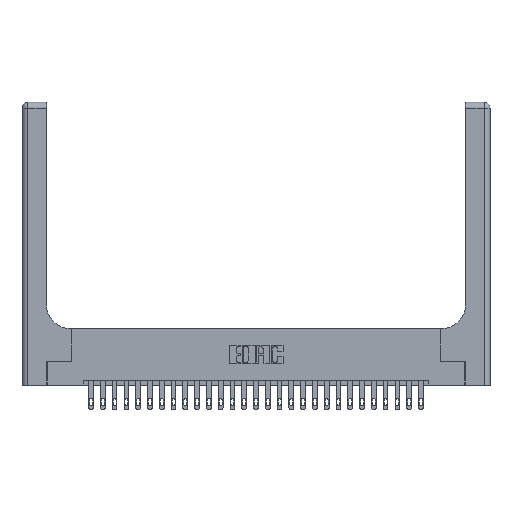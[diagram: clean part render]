
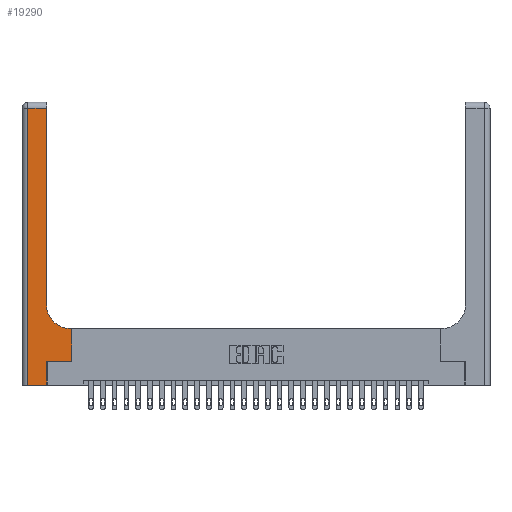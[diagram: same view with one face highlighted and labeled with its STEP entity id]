
A CAD part, top view. The second image highlights one B-rep face of the part: STEP entity #19290.
In plain terms, the highlighted planar face has unit normal (0, 0, 1).
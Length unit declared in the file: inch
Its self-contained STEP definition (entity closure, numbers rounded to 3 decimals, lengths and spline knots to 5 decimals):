
#287 = DIRECTION ( 'NONE',  ( 0., 0., -1. ) ) ;
#476 = EDGE_CURVE ( 'NONE', #22405, #22920, #10577, .T. ) ;
#530 = DIRECTION ( 'NONE',  ( 0., -1., 0. ) ) ;
#1336 = VERTEX_POINT ( 'NONE', #18872 ) ;
#1793 = VERTEX_POINT ( 'NONE', #12462 ) ;
#2691 = VECTOR ( 'NONE', #4734, 39.37008 ) ;
#3200 = CARTESIAN_POINT ( 'NONE',  ( 0.265, 0.25, 0.37 ) ) ;
#4323 = VECTOR ( 'NONE', #20410, 39.37008 ) ;
#4428 = LINE ( 'NONE', #23017, #19224 ) ;
#4638 = DIRECTION ( 'NONE',  ( -1., 0., 0. ) ) ;
#4734 = DIRECTION ( 'NONE',  ( 1., 0., 0. ) ) ;
#4810 = DIRECTION ( 'NONE',  ( -1., 0., 0. ) ) ;
#5131 = VECTOR ( 'NONE', #22413, 39.37008 ) ;
#5267 = EDGE_LOOP ( 'NONE', ( #17801, #13367, #9444, #25422, #22040, #21015, #5720, #16554, #16107 ) ) ;
#5720 = ORIENTED_EDGE ( 'NONE', *, *, #18563, .T. ) ;
#5885 = CARTESIAN_POINT ( 'NONE',  ( 0.51, 0.6, 0.37 ) ) ;
#6040 = DIRECTION ( 'NONE',  ( 0., 1., 0. ) ) ;
#6637 = PLANE ( 'NONE',  #23542 ) ;
#6840 = DIRECTION ( 'NONE',  ( 1., 0., 0. ) ) ;
#7243 = CARTESIAN_POINT ( 'NONE',  ( 0.265, 0.25, 0.37 ) ) ;
#8578 = CARTESIAN_POINT ( 'NONE',  ( 0., 2.94, 0.37 ) ) ;
#8591 = VECTOR ( 'NONE', #530, 39.37008 ) ;
#9444 = ORIENTED_EDGE ( 'NONE', *, *, #16379, .T. ) ;
#10037 = LINE ( 'NONE', #16149, #11757 ) ;
#10207 = AXIS2_PLACEMENT_3D ( 'NONE', #25192, #25063, #6840 ) ;
#10384 = VERTEX_POINT ( 'NONE', #10520 ) ;
#10520 = CARTESIAN_POINT ( 'NONE',  ( 0.06, 0., 0.37 ) ) ;
#10577 = LINE ( 'NONE', #8578, #4323 ) ;
#11757 = VECTOR ( 'NONE', #6040, 39.37008 ) ;
#11845 = VERTEX_POINT ( 'NONE', #3200 ) ;
#12185 = CARTESIAN_POINT ( 'NONE',  ( 0.26, 3., 0.37 ) ) ;
#12462 = CARTESIAN_POINT ( 'NONE',  ( 0.265, 0., 0.37 ) ) ;
#12566 = EDGE_CURVE ( 'NONE', #23044, #22405, #18050, .T. ) ;
#12725 = CARTESIAN_POINT ( 'NONE',  ( 0.06, 2.94, 0.37 ) ) ;
#12739 = LINE ( 'NONE', #14986, #8591 ) ;
#12757 = EDGE_CURVE ( 'NONE', #25190, #23044, #21658, .T. ) ;
#13367 = ORIENTED_EDGE ( 'NONE', *, *, #476, .T. ) ;
#14268 = VECTOR ( 'NONE', #16799, 39.37008 ) ;
#14986 = CARTESIAN_POINT ( 'NONE',  ( 0.06, 3., 0.37 ) ) ;
#15117 = LINE ( 'NONE', #7243, #2691 ) ;
#15426 = EDGE_CURVE ( 'NONE', #11845, #1336, #15117, .T. ) ;
#16107 = ORIENTED_EDGE ( 'NONE', *, *, #12757, .T. ) ;
#16149 = CARTESIAN_POINT ( 'NONE',  ( 0.265, 0., 0.37 ) ) ;
#16379 = EDGE_CURVE ( 'NONE', #22920, #10384, #12739, .T. ) ;
#16554 = ORIENTED_EDGE ( 'NONE', *, *, #17164, .T. ) ;
#16799 = DIRECTION ( 'NONE',  ( 1., 0., 0. ) ) ;
#17164 = EDGE_CURVE ( 'NONE', #21154, #25190, #4428, .T. ) ;
#17166 = VECTOR ( 'NONE', #21677, 39.37008 ) ;
#17801 = ORIENTED_EDGE ( 'NONE', *, *, #12566, .T. ) ;
#18050 = LINE ( 'NONE', #12185, #5131 ) ;
#18563 = EDGE_CURVE ( 'NONE', #1336, #21154, #21427, .T. ) ;
#18615 = CARTESIAN_POINT ( 'NONE',  ( 0.26, 2.94, 0.37 ) ) ;
#18872 = CARTESIAN_POINT ( 'NONE',  ( 0.528, 0.25, 0.37 ) ) ;
#19224 = VECTOR ( 'NONE', #4810, 39.37008 ) ;
#19290 = ADVANCED_FACE ( 'NONE', ( #24841 ), #6637, .F. ) ;
#20362 = EDGE_CURVE ( 'NONE', #10384, #1793, #24509, .T. ) ;
#20410 = DIRECTION ( 'NONE',  ( -1., 0., 0. ) ) ;
#20441 = CARTESIAN_POINT ( 'NONE',  ( 0.528, 0.6, 0.37 ) ) ;
#21015 = ORIENTED_EDGE ( 'NONE', *, *, #15426, .T. ) ;
#21154 = VERTEX_POINT ( 'NONE', #20441 ) ;
#21427 = LINE ( 'NONE', #25695, #17166 ) ;
#21658 = CIRCLE ( 'NONE', #10207, 0.25 ) ;
#21677 = DIRECTION ( 'NONE',  ( 0., 1., 0. ) ) ;
#22040 = ORIENTED_EDGE ( 'NONE', *, *, #23774, .T. ) ;
#22405 = VERTEX_POINT ( 'NONE', #18615 ) ;
#22413 = DIRECTION ( 'NONE',  ( 0., 1., 0. ) ) ;
#22767 = CARTESIAN_POINT ( 'NONE',  ( 0., 0., 0.37 ) ) ;
#22845 = CARTESIAN_POINT ( 'NONE',  ( 0., 3., 0.37 ) ) ;
#22920 = VERTEX_POINT ( 'NONE', #12725 ) ;
#23017 = CARTESIAN_POINT ( 'NONE',  ( 0.26, 0.6, 0.37 ) ) ;
#23044 = VERTEX_POINT ( 'NONE', #23587 ) ;
#23542 = AXIS2_PLACEMENT_3D ( 'NONE', #22845, #287, #4638 ) ;
#23587 = CARTESIAN_POINT ( 'NONE',  ( 0.26, 0.85, 0.37 ) ) ;
#23774 = EDGE_CURVE ( 'NONE', #1793, #11845, #10037, .T. ) ;
#24509 = LINE ( 'NONE', #22767, #14268 ) ;
#24841 = FACE_OUTER_BOUND ( 'NONE', #5267, .T. ) ;
#25063 = DIRECTION ( 'NONE',  ( 0., 0., -1. ) ) ;
#25190 = VERTEX_POINT ( 'NONE', #5885 ) ;
#25192 = CARTESIAN_POINT ( 'NONE',  ( 0.51, 0.85, 0.37 ) ) ;
#25422 = ORIENTED_EDGE ( 'NONE', *, *, #20362, .T. ) ;
#25695 = CARTESIAN_POINT ( 'NONE',  ( 0.528, 0.25, 0.37 ) ) ;
